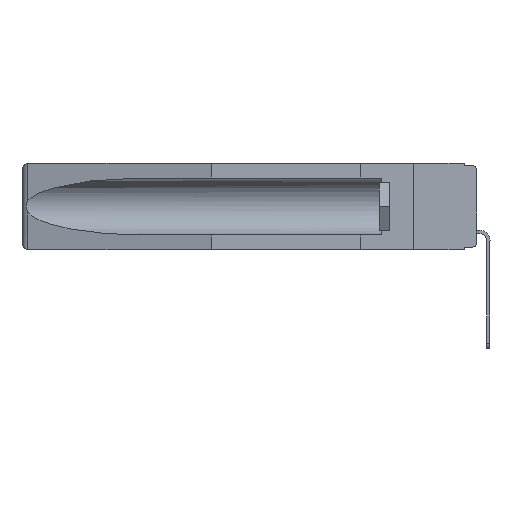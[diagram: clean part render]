
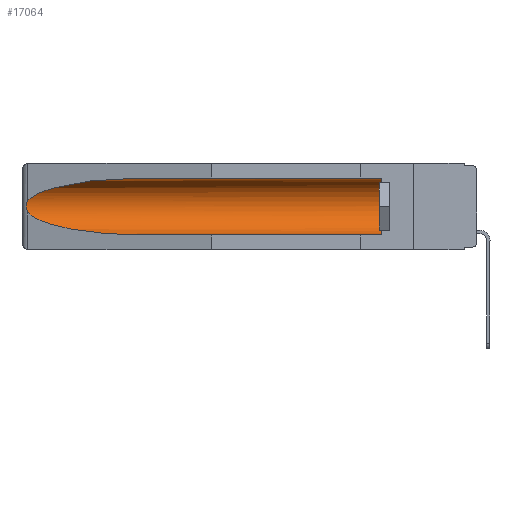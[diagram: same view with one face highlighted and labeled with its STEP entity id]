
A CAD part, left-side view. The second image highlights one B-rep face of the part: STEP entity #17064.
In plain terms, the highlighted cylindrical face has radius 2.857 mm (diameter 5.715 mm), a partial arc.
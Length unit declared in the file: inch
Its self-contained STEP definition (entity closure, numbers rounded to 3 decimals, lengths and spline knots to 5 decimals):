
#78 = CARTESIAN_POINT ( 'NONE',  ( 0.2673, 1.5327, -0.16383 ) ) ;
#115 = EDGE_CURVE ( 'NONE', #7596, #3313, #5226, .T. ) ;
#196 = CARTESIAN_POINT ( 'NONE',  ( 0.2673, 1.53269, -0.17917 ) ) ;
#1128 = CARTESIAN_POINT ( 'NONE',  ( 0.25451, 1.48313, -0.09465 ) ) ;
#1190 = CARTESIAN_POINT ( 'NONE',  ( 0.26537, 1.52718, -0.14972 ) ) ;
#1247 = CARTESIAN_POINT ( 'NONE',  ( 0.26537, 1.52718, -0.14972 ) ) ;
#1874 = VERTEX_POINT ( 'NONE', #10060 ) ;
#2405 =( BOUNDED_CURVE ( )  B_SPLINE_CURVE ( 3, ( #5616, #15883, #1128, #1247 ),
 .UNSPECIFIED., .F., .F. ) 
 B_SPLINE_CURVE_WITH_KNOTS ( ( 4, 4 ),
 ( 4.71239, 6.08839 ),
 .UNSPECIFIED. ) 
 CURVE ( )  GEOMETRIC_REPRESENTATION_ITEM ( )  RATIONAL_B_SPLINE_CURVE ( ( 1., 0.848, 0.848, 1. ) ) 
 REPRESENTATION_ITEM ( '' )  );
#2732 = CARTESIAN_POINT ( 'NONE',  ( 0.155, 0.126, -0.1715 ) ) ;
#2878 = CARTESIAN_POINT ( 'NONE',  ( 0.26537, 1.52718, -0.19328 ) ) ;
#3287 = ORIENTED_EDGE ( 'NONE', *, *, #15173, .T. ) ;
#3313 = VERTEX_POINT ( 'NONE', #8104 ) ;
#3848 = ORIENTED_EDGE ( 'NONE', *, *, #11954, .T. ) ;
#4042 = CARTESIAN_POINT ( 'NONE',  ( 0.25451, 1.48313, -0.24835 ) ) ;
#4858 = AXIS2_PLACEMENT_3D ( 'NONE', #12971, #10197, #13038 ) ;
#5226 = LINE ( 'NONE', #12637, #14516 ) ;
#5616 = CARTESIAN_POINT ( 'NONE',  ( 0.155, 1.07973, -0.059 ) ) ;
#6339 = ORIENTED_EDGE ( 'NONE', *, *, #7280, .T. ) ;
#7095 = DIRECTION ( 'NONE',  ( 0., 0., 1. ) ) ;
#7280 = EDGE_CURVE ( 'NONE', #9914, #11808, #2405, .T. ) ;
#7596 = VERTEX_POINT ( 'NONE', #8810 ) ;
#8104 = CARTESIAN_POINT ( 'NONE',  ( 0.155, 1.07973, -0.284 ) ) ;
#8270 = CIRCLE ( 'NONE', #16840, 0.1125 ) ;
#8480 = LINE ( 'NONE', #10593, #14572 ) ;
#8601 = EDGE_CURVE ( 'NONE', #11808, #11238, #18405, .T. ) ;
#8810 = CARTESIAN_POINT ( 'NONE',  ( 0.155, 0.126, -0.284 ) ) ;
#9914 = VERTEX_POINT ( 'NONE', #18775 ) ;
#10060 = CARTESIAN_POINT ( 'NONE',  ( 0.155, 0.126, -0.059 ) ) ;
#10197 = DIRECTION ( 'NONE',  ( 0., 1., 0. ) ) ;
#10223 = CARTESIAN_POINT ( 'NONE',  ( 0.26597, 1.52961, -0.15275 ) ) ;
#10593 = CARTESIAN_POINT ( 'NONE',  ( 0.155, -0.30754, -0.059 ) ) ;
#11238 = VERTEX_POINT ( 'NONE', #16360 ) ;
#11284 = CARTESIAN_POINT ( 'NONE',  ( 0.26537, 1.52718, -0.19328 ) ) ;
#11627 = CARTESIAN_POINT ( 'NONE',  ( 0.2675, 1.53308, -0.16763 ) ) ;
#11808 = VERTEX_POINT ( 'NONE', #18241 ) ;
#11815 = CYLINDRICAL_SURFACE ( 'NONE', #4858, 0.1125 ) ;
#11954 = EDGE_CURVE ( 'NONE', #7596, #1874, #8270, .T. ) ;
#12637 = CARTESIAN_POINT ( 'NONE',  ( 0.155, -0.30754, -0.284 ) ) ;
#12826 = DIRECTION ( 'NONE',  ( 0., 1., 0. ) ) ;
#12915 = EDGE_CURVE ( 'NONE', #1874, #9914, #8480, .T. ) ;
#12971 = CARTESIAN_POINT ( 'NONE',  ( 0.155, -0.30754, -0.1715 ) ) ;
#13038 = DIRECTION ( 'NONE',  ( 0., 0., 1. ) ) ;
#13683 = DIRECTION ( 'NONE',  ( 0., 1., 0. ) ) ;
#13848 = FACE_OUTER_BOUND ( 'NONE', #15681, .T. ) ;
#14116 = CARTESIAN_POINT ( 'NONE',  ( 0.155, 1.07973, -0.284 ) ) ;
#14254 =( BOUNDED_CURVE ( )  B_SPLINE_CURVE ( 3, ( #11284, #4042, #17145, #14116 ),
 .UNSPECIFIED., .F., .F. ) 
 B_SPLINE_CURVE_WITH_KNOTS ( ( 4, 4 ),
 ( 0.1948, 1.5708 ),
 .UNSPECIFIED. ) 
 CURVE ( )  GEOMETRIC_REPRESENTATION_ITEM ( )  RATIONAL_B_SPLINE_CURVE ( ( 1., 0.848, 0.848, 1. ) ) 
 REPRESENTATION_ITEM ( '' )  );
#14330 = DIRECTION ( 'NONE',  ( 0., -1., 0. ) ) ;
#14516 = VECTOR ( 'NONE', #12826, 39.37008 ) ;
#14572 = VECTOR ( 'NONE', #13683, 39.37008 ) ;
#14663 = CARTESIAN_POINT ( 'NONE',  ( 0.26655, 1.53094, -0.18657 ) ) ;
#14855 = CARTESIAN_POINT ( 'NONE',  ( 0.26597, 1.5296, -0.19026 ) ) ;
#15173 = EDGE_CURVE ( 'NONE', #11238, #3313, #14254, .T. ) ;
#15563 = CARTESIAN_POINT ( 'NONE',  ( 0.2675, 1.53308, -0.17534 ) ) ;
#15681 = EDGE_LOOP ( 'NONE', ( #6339, #16415, #3287, #18477, #3848, #17823 ) ) ;
#15883 = CARTESIAN_POINT ( 'NONE',  ( 0.21114, 1.30732, -0.059 ) ) ;
#16360 = CARTESIAN_POINT ( 'NONE',  ( 0.26537, 1.52718, -0.19328 ) ) ;
#16415 = ORIENTED_EDGE ( 'NONE', *, *, #8601, .T. ) ;
#16840 = AXIS2_PLACEMENT_3D ( 'NONE', #2732, #14330, #7095 ) ;
#17064 = ADVANCED_FACE ( 'NONE', ( #13848 ), #11815, .F. ) ;
#17145 = CARTESIAN_POINT ( 'NONE',  ( 0.21114, 1.30732, -0.284 ) ) ;
#17620 = CARTESIAN_POINT ( 'NONE',  ( 0.26654, 1.53092, -0.15636 ) ) ;
#17823 = ORIENTED_EDGE ( 'NONE', *, *, #12915, .T. ) ;
#18241 = CARTESIAN_POINT ( 'NONE',  ( 0.26537, 1.52718, -0.14972 ) ) ;
#18405 = B_SPLINE_CURVE_WITH_KNOTS ( 'NONE', 3,
 ( #1190, #10223, #17620, #78, #11627, #15563, #196, #14663, #14855, #2878 ),
 .UNSPECIFIED., .F., .F.,
 ( 4, 2, 2, 2, 4 ),
 ( 0., 0.00029, 0.00058, 0.00087, 0.00117 ),
 .UNSPECIFIED. ) ;
#18477 = ORIENTED_EDGE ( 'NONE', *, *, #115, .F. ) ;
#18775 = CARTESIAN_POINT ( 'NONE',  ( 0.155, 1.07973, -0.059 ) ) ;
